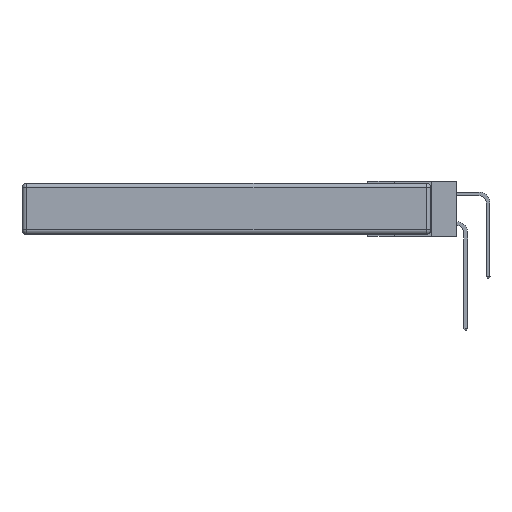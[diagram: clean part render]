
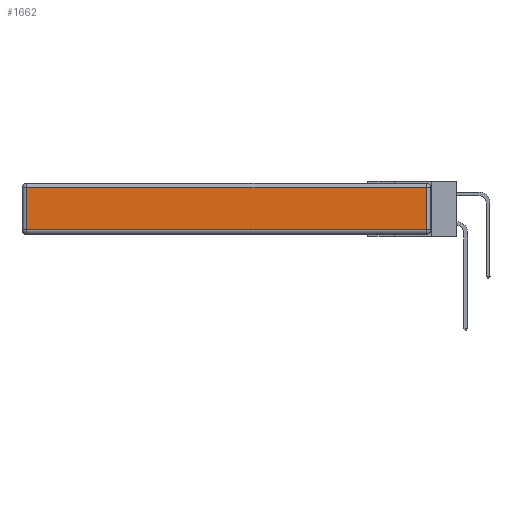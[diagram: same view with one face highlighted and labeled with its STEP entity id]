
A CAD part, left-side view. The second image highlights one B-rep face of the part: STEP entity #1662.
In plain terms, the highlighted planar face has unit normal (-1, 0, 0).
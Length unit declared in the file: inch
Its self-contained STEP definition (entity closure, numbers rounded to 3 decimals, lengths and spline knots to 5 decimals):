
#185 = CARTESIAN_POINT ( 'NONE',  ( 0., 0.03, -0.313 ) ) ;
#229 = PLANE ( 'NONE',  #16760 ) ;
#1662 = ADVANCED_FACE ( 'NONE', ( #9235 ), #229, .T. ) ;
#2231 = LINE ( 'NONE', #17259, #5040 ) ;
#4167 = VERTEX_POINT ( 'NONE', #16592 ) ;
#5033 = EDGE_CURVE ( 'NONE', #20041, #4167, #9251, .T. ) ;
#5040 = VECTOR ( 'NONE', #8231, 39.37008 ) ;
#5205 = ORIENTED_EDGE ( 'NONE', *, *, #15214, .T. ) ;
#6787 = VERTEX_POINT ( 'NONE', #22851 ) ;
#7457 = CARTESIAN_POINT ( 'NONE',  ( 0., 0., -0.343 ) ) ;
#7559 = LINE ( 'NONE', #20512, #15644 ) ;
#8220 = DIRECTION ( 'NONE',  ( 0., 1., 0. ) ) ;
#8231 = DIRECTION ( 'NONE',  ( 0., 0., 1. ) ) ;
#9235 = FACE_OUTER_BOUND ( 'NONE', #19902, .T. ) ;
#9251 = LINE ( 'NONE', #11883, #11486 ) ;
#10132 = EDGE_CURVE ( 'NONE', #4167, #6787, #7559, .T. ) ;
#10306 = EDGE_CURVE ( 'NONE', #14417, #20041, #2231, .T. ) ;
#11486 = VECTOR ( 'NONE', #8220, 39.37008 ) ;
#11564 = DIRECTION ( 'NONE',  ( 0., -1., 0. ) ) ;
#11630 = DIRECTION ( 'NONE',  ( 0., 0., -1. ) ) ;
#11883 = CARTESIAN_POINT ( 'NONE',  ( 0., 2.75, -0.03 ) ) ;
#12223 = ORIENTED_EDGE ( 'NONE', *, *, #5033, .T. ) ;
#13158 = CARTESIAN_POINT ( 'NONE',  ( 0., 0., -0.313 ) ) ;
#13272 = LINE ( 'NONE', #13158, #20762 ) ;
#14417 = VERTEX_POINT ( 'NONE', #185 ) ;
#15214 = EDGE_CURVE ( 'NONE', #6787, #14417, #13272, .T. ) ;
#15644 = VECTOR ( 'NONE', #11630, 39.37008 ) ;
#15801 = CARTESIAN_POINT ( 'NONE',  ( 0., 0.03, -0.03 ) ) ;
#16281 = DIRECTION ( 'NONE',  ( 0., 0., 1. ) ) ;
#16592 = CARTESIAN_POINT ( 'NONE',  ( 0., 2.72, -0.03 ) ) ;
#16760 = AXIS2_PLACEMENT_3D ( 'NONE', #7457, #21626, #16281 ) ;
#17259 = CARTESIAN_POINT ( 'NONE',  ( 0., 0.03, -0.343 ) ) ;
#19902 = EDGE_LOOP ( 'NONE', ( #5205, #20086, #12223, #21950 ) ) ;
#20041 = VERTEX_POINT ( 'NONE', #15801 ) ;
#20086 = ORIENTED_EDGE ( 'NONE', *, *, #10306, .T. ) ;
#20512 = CARTESIAN_POINT ( 'NONE',  ( 0., 2.72, -0.343 ) ) ;
#20762 = VECTOR ( 'NONE', #11564, 39.37008 ) ;
#21626 = DIRECTION ( 'NONE',  ( -1., 0., 0. ) ) ;
#21950 = ORIENTED_EDGE ( 'NONE', *, *, #10132, .T. ) ;
#22851 = CARTESIAN_POINT ( 'NONE',  ( 0., 2.72, -0.313 ) ) ;
